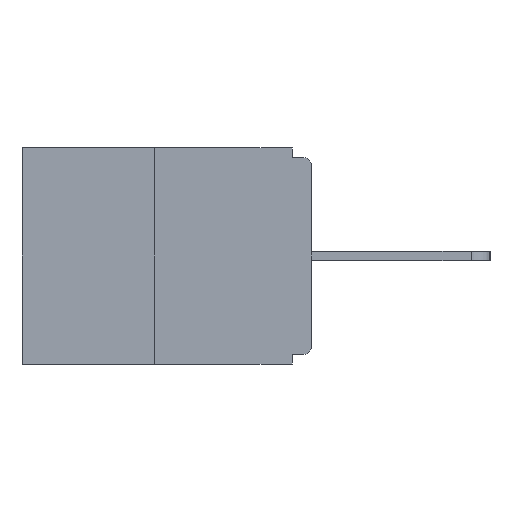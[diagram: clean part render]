
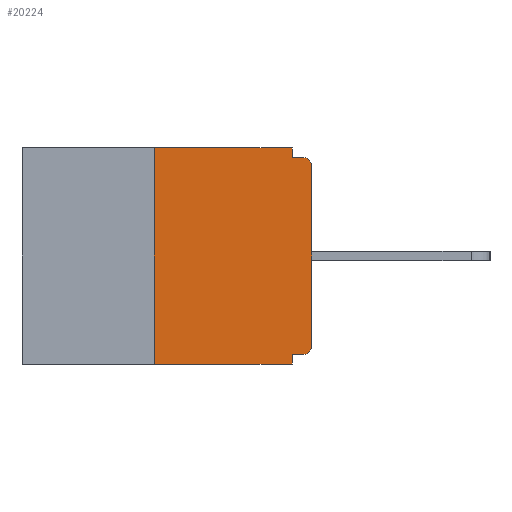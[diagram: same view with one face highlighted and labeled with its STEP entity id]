
A CAD part, left-side view. The second image highlights one B-rep face of the part: STEP entity #20224.
In plain terms, the highlighted planar face has unit normal (-1, 0, 0).
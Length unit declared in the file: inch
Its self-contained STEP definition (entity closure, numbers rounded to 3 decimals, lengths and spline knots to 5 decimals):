
#350 = VECTOR ( 'NONE', #9330, 39.37008 ) ;
#753 = CARTESIAN_POINT ( 'NONE',  ( 0., 0.015, -0.015 ) ) ;
#757 = EDGE_CURVE ( 'NONE', #8077, #6568, #6226, .T. ) ;
#1213 = CARTESIAN_POINT ( 'NONE',  ( 0., 0.25, -0.343 ) ) ;
#1215 = VERTEX_POINT ( 'NONE', #7931 ) ;
#2053 = CARTESIAN_POINT ( 'NONE',  ( 0., 0., -0.313 ) ) ;
#2251 = EDGE_CURVE ( 'NONE', #5488, #11216, #3844, .T. ) ;
#2427 = AXIS2_PLACEMENT_3D ( 'NONE', #23757, #6786, #12461 ) ;
#2579 = DIRECTION ( 'NONE',  ( 1., 0., 0. ) ) ;
#3328 = VERTEX_POINT ( 'NONE', #5591 ) ;
#3786 = CARTESIAN_POINT ( 'NONE',  ( 0., 0.25, 0. ) ) ;
#3844 = LINE ( 'NONE', #9764, #8024 ) ;
#4142 = VERTEX_POINT ( 'NONE', #8823 ) ;
#4419 = CARTESIAN_POINT ( 'NONE',  ( 0., 0.015, -0.03 ) ) ;
#4832 = VERTEX_POINT ( 'NONE', #13480 ) ;
#4917 = DIRECTION ( 'NONE',  ( 0., 0., -1. ) ) ;
#5364 = CARTESIAN_POINT ( 'NONE',  ( 0., 0., -0.328 ) ) ;
#5488 = VERTEX_POINT ( 'NONE', #1213 ) ;
#5522 = LINE ( 'NONE', #24325, #350 ) ;
#5585 = CIRCLE ( 'NONE', #2427, 0.015 ) ;
#5591 = CARTESIAN_POINT ( 'NONE',  ( 0., 0.031, -0.328 ) ) ;
#5613 = ORIENTED_EDGE ( 'NONE', *, *, #7798, .T. ) ;
#5773 = VECTOR ( 'NONE', #20135, 39.37008 ) ;
#6226 = LINE ( 'NONE', #23439, #11037 ) ;
#6562 = ORIENTED_EDGE ( 'NONE', *, *, #18563, .F. ) ;
#6568 = VERTEX_POINT ( 'NONE', #753 ) ;
#6763 = DIRECTION ( 'NONE',  ( -1., 0., 0. ) ) ;
#6786 = DIRECTION ( 'NONE',  ( -1., 0., 0. ) ) ;
#6889 = DIRECTION ( 'NONE',  ( 0., 0., -1. ) ) ;
#7353 = CARTESIAN_POINT ( 'NONE',  ( 0., 0.031, -0.015 ) ) ;
#7798 = EDGE_CURVE ( 'NONE', #4832, #6568, #8162, .T. ) ;
#7910 = DIRECTION ( 'NONE',  ( 0., -1., 0. ) ) ;
#7931 = CARTESIAN_POINT ( 'NONE',  ( 0., 0.031, 0. ) ) ;
#8024 = VECTOR ( 'NONE', #7910, 39.37008 ) ;
#8077 = VERTEX_POINT ( 'NONE', #7353 ) ;
#8107 = EDGE_LOOP ( 'NONE', ( #6562, #15149, #17786, #24354, #15917, #19902, #9729, #5613, #8890, #10381 ) ) ;
#8162 = CIRCLE ( 'NONE', #12930, 0.015 ) ;
#8427 = EDGE_CURVE ( 'NONE', #24391, #3328, #20342, .T. ) ;
#8506 = DIRECTION ( 'NONE',  ( 0., 0., -1. ) ) ;
#8823 = CARTESIAN_POINT ( 'NONE',  ( 0., 0.25, 0. ) ) ;
#8890 = ORIENTED_EDGE ( 'NONE', *, *, #757, .F. ) ;
#9330 = DIRECTION ( 'NONE',  ( 0., 0., 1. ) ) ;
#9729 = ORIENTED_EDGE ( 'NONE', *, *, #10549, .T. ) ;
#9764 = CARTESIAN_POINT ( 'NONE',  ( 0., 0.46, -0.343 ) ) ;
#10381 = ORIENTED_EDGE ( 'NONE', *, *, #14448, .F. ) ;
#10549 = EDGE_CURVE ( 'NONE', #18792, #4832, #5522, .T. ) ;
#11037 = VECTOR ( 'NONE', #12162, 39.37008 ) ;
#11216 = VERTEX_POINT ( 'NONE', #17961 ) ;
#11577 = LINE ( 'NONE', #3786, #23339 ) ;
#12162 = DIRECTION ( 'NONE',  ( 0., -1., 0. ) ) ;
#12461 = DIRECTION ( 'NONE',  ( 0., 0., -1. ) ) ;
#12537 = EDGE_CURVE ( 'NONE', #5488, #4142, #11577, .T. ) ;
#12627 = CARTESIAN_POINT ( 'NONE',  ( 0., 0.015, -0.328 ) ) ;
#12930 = AXIS2_PLACEMENT_3D ( 'NONE', #4419, #6763, #4917 ) ;
#13033 = DIRECTION ( 'NONE',  ( 0., 1., 0. ) ) ;
#13480 = CARTESIAN_POINT ( 'NONE',  ( 0., 0., -0.03 ) ) ;
#13852 = VECTOR ( 'NONE', #6889, 39.37008 ) ;
#14199 = CARTESIAN_POINT ( 'NONE',  ( 0., 0.031, 0. ) ) ;
#14448 = EDGE_CURVE ( 'NONE', #1215, #8077, #20281, .T. ) ;
#14594 = EDGE_CURVE ( 'NONE', #24391, #18792, #5585, .T. ) ;
#14888 = LINE ( 'NONE', #16755, #24101 ) ;
#15149 = ORIENTED_EDGE ( 'NONE', *, *, #12537, .F. ) ;
#15829 = PLANE ( 'NONE',  #19680 ) ;
#15917 = ORIENTED_EDGE ( 'NONE', *, *, #8427, .F. ) ;
#16755 = CARTESIAN_POINT ( 'NONE',  ( 0., 0.031, -0.343 ) ) ;
#17786 = ORIENTED_EDGE ( 'NONE', *, *, #2251, .T. ) ;
#17961 = CARTESIAN_POINT ( 'NONE',  ( 0., 0.031, -0.343 ) ) ;
#18563 = EDGE_CURVE ( 'NONE', #4142, #1215, #23579, .T. ) ;
#18792 = VERTEX_POINT ( 'NONE', #2053 ) ;
#18888 = VECTOR ( 'NONE', #13033, 39.37008 ) ;
#19680 = AXIS2_PLACEMENT_3D ( 'NONE', #21781, #2579, #8506 ) ;
#19902 = ORIENTED_EDGE ( 'NONE', *, *, #14594, .T. ) ;
#20135 = DIRECTION ( 'NONE',  ( 0., -1., 0. ) ) ;
#20224 = ADVANCED_FACE ( 'NONE', ( #23768 ), #15829, .F. ) ;
#20281 = LINE ( 'NONE', #14199, #13852 ) ;
#20342 = LINE ( 'NONE', #5364, #18888 ) ;
#20637 = DIRECTION ( 'NONE',  ( 0., 0., 1. ) ) ;
#21591 = EDGE_CURVE ( 'NONE', #3328, #11216, #14888, .T. ) ;
#21781 = CARTESIAN_POINT ( 'NONE',  ( 0., 0.46, 0. ) ) ;
#23339 = VECTOR ( 'NONE', #20637, 39.37008 ) ;
#23439 = CARTESIAN_POINT ( 'NONE',  ( 0., 0., -0.015 ) ) ;
#23579 = LINE ( 'NONE', #23724, #5773 ) ;
#23724 = CARTESIAN_POINT ( 'NONE',  ( 0., 0.46, 0. ) ) ;
#23757 = CARTESIAN_POINT ( 'NONE',  ( 0., 0.015, -0.313 ) ) ;
#23768 = FACE_OUTER_BOUND ( 'NONE', #8107, .T. ) ;
#24101 = VECTOR ( 'NONE', #24315, 39.37008 ) ;
#24315 = DIRECTION ( 'NONE',  ( 0., 0., -1. ) ) ;
#24325 = CARTESIAN_POINT ( 'NONE',  ( 0., 0., 0. ) ) ;
#24354 = ORIENTED_EDGE ( 'NONE', *, *, #21591, .F. ) ;
#24391 = VERTEX_POINT ( 'NONE', #12627 ) ;
